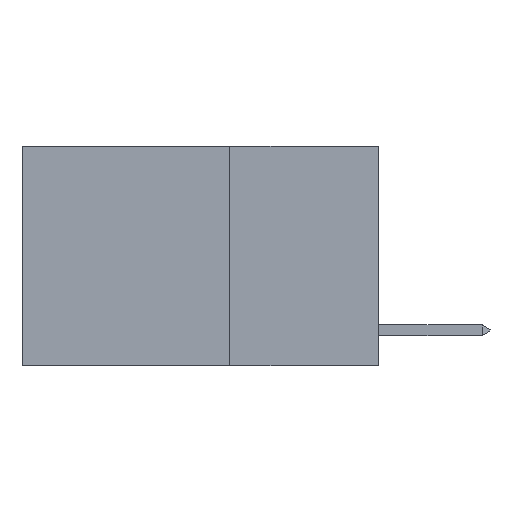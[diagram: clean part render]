
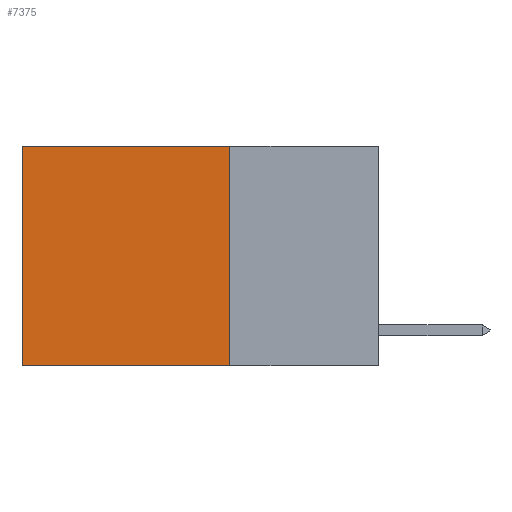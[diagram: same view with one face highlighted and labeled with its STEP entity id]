
A CAD part, left-side view. The second image highlights one B-rep face of the part: STEP entity #7375.
In plain terms, the highlighted planar face has unit normal (-1, 0, 0).
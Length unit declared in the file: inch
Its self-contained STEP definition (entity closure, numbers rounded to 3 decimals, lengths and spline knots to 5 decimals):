
#347 = DIRECTION ( 'NONE',  ( 0., 0., -1. ) ) ;
#404 = VECTOR ( 'NONE', #347, 39.37008 ) ;
#420 = PLANE ( 'NONE',  #4991 ) ;
#1487 = VERTEX_POINT ( 'NONE', #10028 ) ;
#1540 = EDGE_CURVE ( 'NONE', #6586, #1487, #2953, .T. ) ;
#1556 = EDGE_CURVE ( 'NONE', #1487, #1580, #6927, .T. ) ;
#1580 = VERTEX_POINT ( 'NONE', #4693 ) ;
#2310 = CARTESIAN_POINT ( 'NONE',  ( 0.2625, 0.25, 0. ) ) ;
#2703 = VECTOR ( 'NONE', #6894, 39.37008 ) ;
#2953 = LINE ( 'NONE', #3596, #2703 ) ;
#3596 = CARTESIAN_POINT ( 'NONE',  ( 0.2625, 0.25, 0. ) ) ;
#3637 = ORIENTED_EDGE ( 'NONE', *, *, #8566, .F. ) ;
#3899 = LINE ( 'NONE', #6279, #9934 ) ;
#4453 = ORIENTED_EDGE ( 'NONE', *, *, #1540, .T. ) ;
#4676 = DIRECTION ( 'NONE',  ( 0., 1., 0. ) ) ;
#4679 = VERTEX_POINT ( 'NONE', #6123 ) ;
#4693 = CARTESIAN_POINT ( 'NONE',  ( 0.2625, 0.6, -0.37 ) ) ;
#4991 = AXIS2_PLACEMENT_3D ( 'NONE', #6996, #8695, #6231 ) ;
#5000 = EDGE_CURVE ( 'NONE', #4679, #1580, #3899, .T. ) ;
#5580 = CARTESIAN_POINT ( 'NONE',  ( 0.2625, 0.25, 0. ) ) ;
#6095 = EDGE_LOOP ( 'NONE', ( #7923, #6276, #3637, #4453 ) ) ;
#6123 = CARTESIAN_POINT ( 'NONE',  ( 0.2625, 0.25, -0.37 ) ) ;
#6231 = DIRECTION ( 'NONE',  ( 0., 0., -1. ) ) ;
#6276 = ORIENTED_EDGE ( 'NONE', *, *, #5000, .F. ) ;
#6277 = VECTOR ( 'NONE', #8916, 39.37008 ) ;
#6279 = CARTESIAN_POINT ( 'NONE',  ( 0.2625, 0.25, -0.37 ) ) ;
#6436 = FACE_OUTER_BOUND ( 'NONE', #6095, .T. ) ;
#6586 = VERTEX_POINT ( 'NONE', #5580 ) ;
#6894 = DIRECTION ( 'NONE',  ( 0., 1., 0. ) ) ;
#6927 = LINE ( 'NONE', #8651, #404 ) ;
#6996 = CARTESIAN_POINT ( 'NONE',  ( 0.2625, 0.25, 0. ) ) ;
#7375 = ADVANCED_FACE ( 'NONE', ( #6436 ), #420, .F. ) ;
#7923 = ORIENTED_EDGE ( 'NONE', *, *, #1556, .T. ) ;
#8566 = EDGE_CURVE ( 'NONE', #6586, #4679, #8989, .T. ) ;
#8651 = CARTESIAN_POINT ( 'NONE',  ( 0.2625, 0.6, 0. ) ) ;
#8695 = DIRECTION ( 'NONE',  ( 1., 0., 0. ) ) ;
#8916 = DIRECTION ( 'NONE',  ( 0., 0., -1. ) ) ;
#8989 = LINE ( 'NONE', #2310, #6277 ) ;
#9934 = VECTOR ( 'NONE', #4676, 39.37008 ) ;
#10028 = CARTESIAN_POINT ( 'NONE',  ( 0.2625, 0.6, 0. ) ) ;
